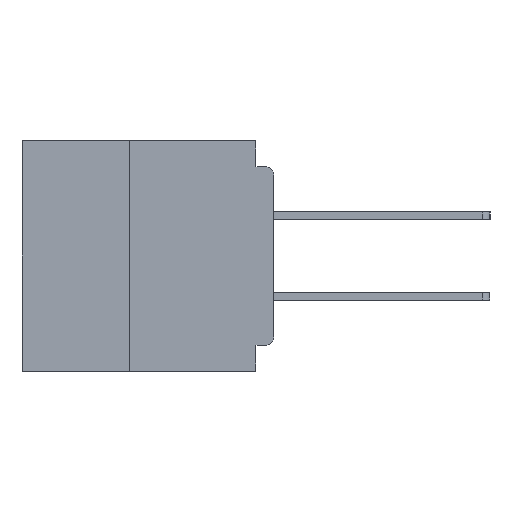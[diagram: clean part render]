
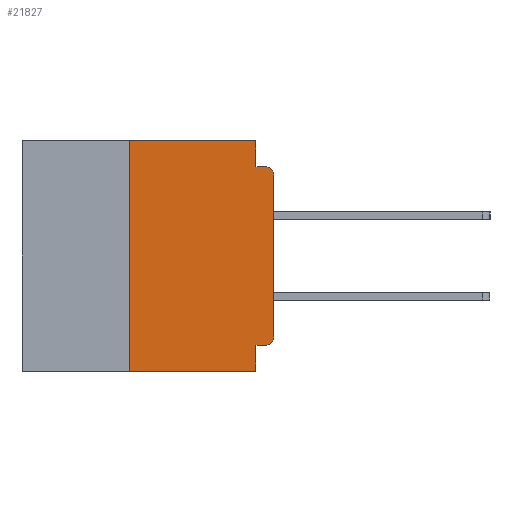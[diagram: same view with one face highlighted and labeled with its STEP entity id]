
A CAD part, left-side view. The second image highlights one B-rep face of the part: STEP entity #21827.
In plain terms, the highlighted planar face has unit normal (-1, 0, 0).
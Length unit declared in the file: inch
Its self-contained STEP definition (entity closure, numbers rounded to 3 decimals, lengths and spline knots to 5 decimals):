
#29 = EDGE_CURVE ( 'NONE', #9606, #14379, #26468, .T. ) ;
#479 = DIRECTION ( 'NONE',  ( 0., -1., 0. ) ) ;
#677 = DIRECTION ( 'NONE',  ( 0., 0., 1. ) ) ;
#1459 = ORIENTED_EDGE ( 'NONE', *, *, #22447, .T. ) ;
#1925 = CARTESIAN_POINT ( 'NONE',  ( 0., 0.031, -0.4 ) ) ;
#2991 = EDGE_CURVE ( 'NONE', #35112, #24631, #34629, .T. ) ;
#3425 = PLANE ( 'NONE',  #18108 ) ;
#3619 = LINE ( 'NONE', #11904, #33144 ) ;
#3709 = LINE ( 'NONE', #19353, #11411 ) ;
#4499 = VECTOR ( 'NONE', #22805, 39.37008 ) ;
#5452 = DIRECTION ( 'NONE',  ( -1., 0., 0. ) ) ;
#6655 = CARTESIAN_POINT ( 'NONE',  ( 0., 0.031, -0.355 ) ) ;
#7522 = ORIENTED_EDGE ( 'NONE', *, *, #26370, .F. ) ;
#7761 = EDGE_CURVE ( 'NONE', #25227, #11218, #24341, .T. ) ;
#7983 = CARTESIAN_POINT ( 'NONE',  ( 0., 0.015, -0.045 ) ) ;
#8627 = EDGE_CURVE ( 'NONE', #14110, #36534, #31840, .T. ) ;
#9154 = CARTESIAN_POINT ( 'NONE',  ( 0., 0.437, 0. ) ) ;
#9606 = VERTEX_POINT ( 'NONE', #12837 ) ;
#10120 = EDGE_CURVE ( 'NONE', #14110, #12816, #29554, .T. ) ;
#10225 = EDGE_CURVE ( 'NONE', #12816, #11218, #34295, .T. ) ;
#10484 = VECTOR ( 'NONE', #677, 39.37008 ) ;
#11132 = DIRECTION ( 'NONE',  ( 0., -1., 0. ) ) ;
#11218 = VERTEX_POINT ( 'NONE', #1925 ) ;
#11376 = ORIENTED_EDGE ( 'NONE', *, *, #10120, .F. ) ;
#11411 = VECTOR ( 'NONE', #36189, 39.37008 ) ;
#11630 = EDGE_CURVE ( 'NONE', #14379, #24631, #11858, .T. ) ;
#11858 = LINE ( 'NONE', #20921, #19503 ) ;
#11904 = CARTESIAN_POINT ( 'NONE',  ( 0., 0.437, 0. ) ) ;
#12099 = ORIENTED_EDGE ( 'NONE', *, *, #13368, .F. ) ;
#12165 = DIRECTION ( 'NONE',  ( 0., 0., -1. ) ) ;
#12816 = VERTEX_POINT ( 'NONE', #6655 ) ;
#12817 = CARTESIAN_POINT ( 'NONE',  ( 0., 0.437, -0.4 ) ) ;
#12837 = CARTESIAN_POINT ( 'NONE',  ( 0., 0.031, 0. ) ) ;
#13368 = EDGE_CURVE ( 'NONE', #20629, #9606, #3619, .T. ) ;
#14110 = VERTEX_POINT ( 'NONE', #18791 ) ;
#14320 = VECTOR ( 'NONE', #29956, 39.37008 ) ;
#14379 = VERTEX_POINT ( 'NONE', #17036 ) ;
#15866 = VECTOR ( 'NONE', #11132, 39.37008 ) ;
#15942 = FACE_OUTER_BOUND ( 'NONE', #22423, .T. ) ;
#16867 = CARTESIAN_POINT ( 'NONE',  ( 0., 0.25, -0.4 ) ) ;
#17036 = CARTESIAN_POINT ( 'NONE',  ( 0., 0.031, -0.045 ) ) ;
#18108 = AXIS2_PLACEMENT_3D ( 'NONE', #9154, #29294, #12165 ) ;
#18791 = CARTESIAN_POINT ( 'NONE',  ( 0., 0.015, -0.355 ) ) ;
#19280 = VECTOR ( 'NONE', #32949, 39.37008 ) ;
#19353 = CARTESIAN_POINT ( 'NONE',  ( 0., 0.25, -0.4 ) ) ;
#19503 = VECTOR ( 'NONE', #34947, 39.37008 ) ;
#20629 = VERTEX_POINT ( 'NONE', #29639 ) ;
#20921 = CARTESIAN_POINT ( 'NONE',  ( 0., 0., -0.045 ) ) ;
#21827 = ADVANCED_FACE ( 'NONE', ( #15942 ), #3425, .F. ) ;
#22423 = EDGE_LOOP ( 'NONE', ( #1459, #33334, #28514, #32613, #12099, #7522, #24716, #30362, #11376, #24983 ) ) ;
#22447 = EDGE_CURVE ( 'NONE', #36534, #35112, #33199, .T. ) ;
#22659 = CARTESIAN_POINT ( 'NONE',  ( 0., 0.015, -0.34 ) ) ;
#22805 = DIRECTION ( 'NONE',  ( 0., 0., -1. ) ) ;
#22812 = CARTESIAN_POINT ( 'NONE',  ( 0., 0.031, 0. ) ) ;
#23108 = DIRECTION ( 'NONE',  ( 0., 0., -1. ) ) ;
#23183 = DIRECTION ( 'NONE',  ( -1., 0., 0. ) ) ;
#23221 = CARTESIAN_POINT ( 'NONE',  ( 0., 0.015, -0.06 ) ) ;
#24167 = CARTESIAN_POINT ( 'NONE',  ( 0., 0., -0.06 ) ) ;
#24222 = AXIS2_PLACEMENT_3D ( 'NONE', #22659, #5452, #25523 ) ;
#24341 = LINE ( 'NONE', #12817, #15866 ) ;
#24631 = VERTEX_POINT ( 'NONE', #7983 ) ;
#24716 = ORIENTED_EDGE ( 'NONE', *, *, #7761, .T. ) ;
#24983 = ORIENTED_EDGE ( 'NONE', *, *, #8627, .T. ) ;
#25227 = VERTEX_POINT ( 'NONE', #16867 ) ;
#25523 = DIRECTION ( 'NONE',  ( 0., 0., -1. ) ) ;
#26370 = EDGE_CURVE ( 'NONE', #25227, #20629, #3709, .T. ) ;
#26468 = LINE ( 'NONE', #22812, #4499 ) ;
#28514 = ORIENTED_EDGE ( 'NONE', *, *, #11630, .F. ) ;
#29294 = DIRECTION ( 'NONE',  ( 1., 0., 0. ) ) ;
#29554 = LINE ( 'NONE', #35328, #14320 ) ;
#29639 = CARTESIAN_POINT ( 'NONE',  ( 0., 0.25, 0. ) ) ;
#29956 = DIRECTION ( 'NONE',  ( 0., 1., 0. ) ) ;
#30362 = ORIENTED_EDGE ( 'NONE', *, *, #10225, .F. ) ;
#31840 = CIRCLE ( 'NONE', #24222, 0.015 ) ;
#32613 = ORIENTED_EDGE ( 'NONE', *, *, #29, .F. ) ;
#32949 = DIRECTION ( 'NONE',  ( 0., 0., -1. ) ) ;
#33144 = VECTOR ( 'NONE', #479, 39.37008 ) ;
#33192 = CARTESIAN_POINT ( 'NONE',  ( 0., 0.031, -0.4 ) ) ;
#33199 = LINE ( 'NONE', #34910, #10484 ) ;
#33300 = AXIS2_PLACEMENT_3D ( 'NONE', #23221, #23183, #23108 ) ;
#33334 = ORIENTED_EDGE ( 'NONE', *, *, #2991, .T. ) ;
#34295 = LINE ( 'NONE', #33192, #19280 ) ;
#34629 = CIRCLE ( 'NONE', #33300, 0.015 ) ;
#34910 = CARTESIAN_POINT ( 'NONE',  ( 0., 0., 0. ) ) ;
#34947 = DIRECTION ( 'NONE',  ( 0., -1., 0. ) ) ;
#35112 = VERTEX_POINT ( 'NONE', #24167 ) ;
#35328 = CARTESIAN_POINT ( 'NONE',  ( 0., 0., -0.355 ) ) ;
#36185 = CARTESIAN_POINT ( 'NONE',  ( 0., 0., -0.34 ) ) ;
#36189 = DIRECTION ( 'NONE',  ( 0., 0., 1. ) ) ;
#36534 = VERTEX_POINT ( 'NONE', #36185 ) ;
